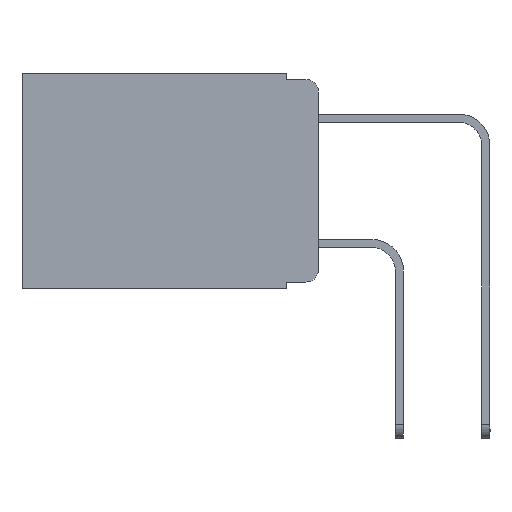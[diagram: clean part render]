
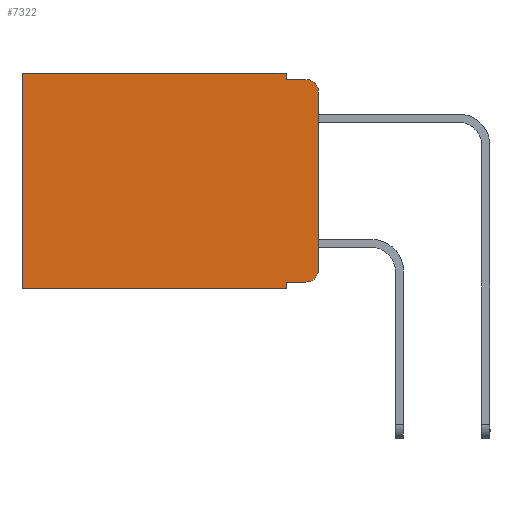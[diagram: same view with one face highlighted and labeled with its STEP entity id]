
A CAD part, left-side view. The second image highlights one B-rep face of the part: STEP entity #7322.
In plain terms, the highlighted planar face has unit normal (-1, 0, 0).
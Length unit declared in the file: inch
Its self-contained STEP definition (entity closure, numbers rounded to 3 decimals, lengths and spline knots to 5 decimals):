
#75 = LINE ( 'NONE', #7190, #1820 ) ;
#102 = VERTEX_POINT ( 'NONE', #17338 ) ;
#327 = EDGE_LOOP ( 'NONE', ( #15962, #14608, #11343, #8410, #2766, #3100, #5046, #13242, #4755, #13850 ) ) ;
#392 = CIRCLE ( 'NONE', #11643, 0.02 ) ;
#913 = VERTEX_POINT ( 'NONE', #10220 ) ;
#1366 = DIRECTION ( 'NONE',  ( 1., 0., 0. ) ) ;
#1820 = VECTOR ( 'NONE', #16833, 39.37008 ) ;
#1852 = VERTEX_POINT ( 'NONE', #7891 ) ;
#2244 = VECTOR ( 'NONE', #6377, 39.37008 ) ;
#2314 = LINE ( 'NONE', #9640, #16110 ) ;
#2385 = VERTEX_POINT ( 'NONE', #4919 ) ;
#2442 = DIRECTION ( 'NONE',  ( 0., 0., -1. ) ) ;
#2642 = CARTESIAN_POINT ( 'NONE',  ( 0.298, 0.051, -0.01 ) ) ;
#2687 = PLANE ( 'NONE',  #9875 ) ;
#2691 = VECTOR ( 'NONE', #12289, 39.37008 ) ;
#2766 = ORIENTED_EDGE ( 'NONE', *, *, #11448, .T. ) ;
#3100 = ORIENTED_EDGE ( 'NONE', *, *, #4786, .T. ) ;
#3251 = EDGE_CURVE ( 'NONE', #12461, #13335, #392, .T. ) ;
#3358 = CARTESIAN_POINT ( 'NONE',  ( 0.298, 0.051, -0.333 ) ) ;
#3382 = CIRCLE ( 'NONE', #6693, 0.02 ) ;
#3917 = CARTESIAN_POINT ( 'NONE',  ( 0.298, 0.051, -0.343 ) ) ;
#4075 = VECTOR ( 'NONE', #2442, 39.37008 ) ;
#4130 = EDGE_CURVE ( 'NONE', #7950, #9368, #2314, .T. ) ;
#4755 = ORIENTED_EDGE ( 'NONE', *, *, #13834, .T. ) ;
#4786 = EDGE_CURVE ( 'NONE', #102, #9368, #16407, .T. ) ;
#4818 = CARTESIAN_POINT ( 'NONE',  ( 0.298, 0.051, -0.333 ) ) ;
#4919 = CARTESIAN_POINT ( 'NONE',  ( 0.298, 0., -0.03 ) ) ;
#4989 = CARTESIAN_POINT ( 'NONE',  ( 0.298, 0.02, -0.03 ) ) ;
#4999 = CARTESIAN_POINT ( 'NONE',  ( 0.298, 0., -0.313 ) ) ;
#5046 = ORIENTED_EDGE ( 'NONE', *, *, #4130, .F. ) ;
#5048 = LINE ( 'NONE', #2642, #2691 ) ;
#5286 = VECTOR ( 'NONE', #17276, 39.37008 ) ;
#5964 = CARTESIAN_POINT ( 'NONE',  ( 0.298, 0.02, -0.313 ) ) ;
#6179 = FACE_OUTER_BOUND ( 'NONE', #327, .T. ) ;
#6377 = DIRECTION ( 'NONE',  ( 0., -1., 0. ) ) ;
#6386 = DIRECTION ( 'NONE',  ( -1., 0., 0. ) ) ;
#6693 = AXIS2_PLACEMENT_3D ( 'NONE', #4989, #6386, #16043 ) ;
#6733 = DIRECTION ( 'NONE',  ( 0., 0., -1. ) ) ;
#6830 = VERTEX_POINT ( 'NONE', #4818 ) ;
#6942 = DIRECTION ( 'NONE',  ( 0., 1., 0. ) ) ;
#7190 = CARTESIAN_POINT ( 'NONE',  ( 0.298, 0., 0. ) ) ;
#7228 = CARTESIAN_POINT ( 'NONE',  ( 0.298, 0.051, 0. ) ) ;
#7322 = ADVANCED_FACE ( 'NONE', ( #6179 ), #2687, .F. ) ;
#7891 = CARTESIAN_POINT ( 'NONE',  ( 0.298, 0.051, -0.01 ) ) ;
#7940 = VECTOR ( 'NONE', #16366, 39.37008 ) ;
#7950 = VERTEX_POINT ( 'NONE', #3917 ) ;
#8410 = ORIENTED_EDGE ( 'NONE', *, *, #12602, .F. ) ;
#8648 = VERTEX_POINT ( 'NONE', #12349 ) ;
#8944 = CARTESIAN_POINT ( 'NONE',  ( 0.298, 0.02, -0.333 ) ) ;
#9368 = VERTEX_POINT ( 'NONE', #10575 ) ;
#9640 = CARTESIAN_POINT ( 'NONE',  ( 0.298, 0., -0.343 ) ) ;
#9875 = AXIS2_PLACEMENT_3D ( 'NONE', #15045, #1366, #6733 ) ;
#9999 = DIRECTION ( 'NONE',  ( 0., 0., -1. ) ) ;
#10220 = CARTESIAN_POINT ( 'NONE',  ( 0.298, 0.02, -0.01 ) ) ;
#10575 = CARTESIAN_POINT ( 'NONE',  ( 0.298, 0.473, -0.343 ) ) ;
#10874 = LINE ( 'NONE', #7228, #17339 ) ;
#11343 = ORIENTED_EDGE ( 'NONE', *, *, #14072, .F. ) ;
#11407 = DIRECTION ( 'NONE',  ( -1., 0., 0. ) ) ;
#11448 = EDGE_CURVE ( 'NONE', #8648, #102, #16363, .T. ) ;
#11643 = AXIS2_PLACEMENT_3D ( 'NONE', #5964, #11407, #14043 ) ;
#11747 = LINE ( 'NONE', #3358, #2244 ) ;
#11781 = EDGE_CURVE ( 'NONE', #2385, #913, #3382, .T. ) ;
#12289 = DIRECTION ( 'NONE',  ( 0., -1., 0. ) ) ;
#12349 = CARTESIAN_POINT ( 'NONE',  ( 0.298, 0.051, 0. ) ) ;
#12461 = VERTEX_POINT ( 'NONE', #8944 ) ;
#12602 = EDGE_CURVE ( 'NONE', #8648, #1852, #16320, .T. ) ;
#13222 = CARTESIAN_POINT ( 'NONE',  ( 0.298, 0., 0. ) ) ;
#13242 = ORIENTED_EDGE ( 'NONE', *, *, #13738, .F. ) ;
#13335 = VERTEX_POINT ( 'NONE', #4999 ) ;
#13738 = EDGE_CURVE ( 'NONE', #6830, #7950, #10874, .T. ) ;
#13834 = EDGE_CURVE ( 'NONE', #6830, #12461, #11747, .T. ) ;
#13850 = ORIENTED_EDGE ( 'NONE', *, *, #3251, .T. ) ;
#14043 = DIRECTION ( 'NONE',  ( 0., 0., -1. ) ) ;
#14072 = EDGE_CURVE ( 'NONE', #1852, #913, #5048, .T. ) ;
#14608 = ORIENTED_EDGE ( 'NONE', *, *, #11781, .T. ) ;
#14839 = EDGE_CURVE ( 'NONE', #2385, #13335, #75, .T. ) ;
#15045 = CARTESIAN_POINT ( 'NONE',  ( 0.298, 0., 0. ) ) ;
#15962 = ORIENTED_EDGE ( 'NONE', *, *, #14839, .F. ) ;
#16043 = DIRECTION ( 'NONE',  ( 0., 0., -1. ) ) ;
#16110 = VECTOR ( 'NONE', #6942, 39.37008 ) ;
#16139 = CARTESIAN_POINT ( 'NONE',  ( 0.298, 0.473, 0. ) ) ;
#16142 = CARTESIAN_POINT ( 'NONE',  ( 0.298, 0.051, 0. ) ) ;
#16320 = LINE ( 'NONE', #16142, #5286 ) ;
#16363 = LINE ( 'NONE', #13222, #7940 ) ;
#16366 = DIRECTION ( 'NONE',  ( 0., 1., 0. ) ) ;
#16407 = LINE ( 'NONE', #16139, #4075 ) ;
#16833 = DIRECTION ( 'NONE',  ( 0., 0., -1. ) ) ;
#17276 = DIRECTION ( 'NONE',  ( 0., 0., -1. ) ) ;
#17338 = CARTESIAN_POINT ( 'NONE',  ( 0.298, 0.473, 0. ) ) ;
#17339 = VECTOR ( 'NONE', #9999, 39.37008 ) ;
